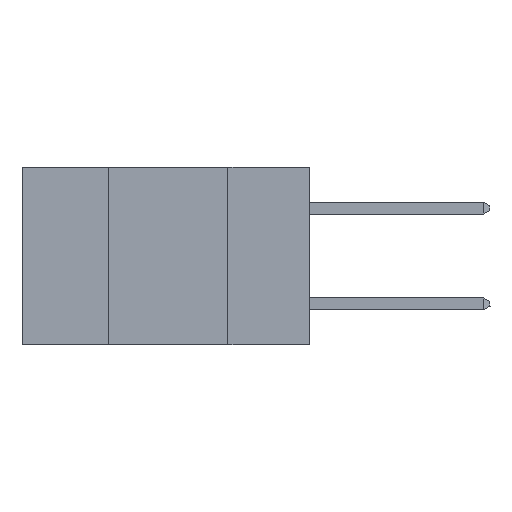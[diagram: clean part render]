
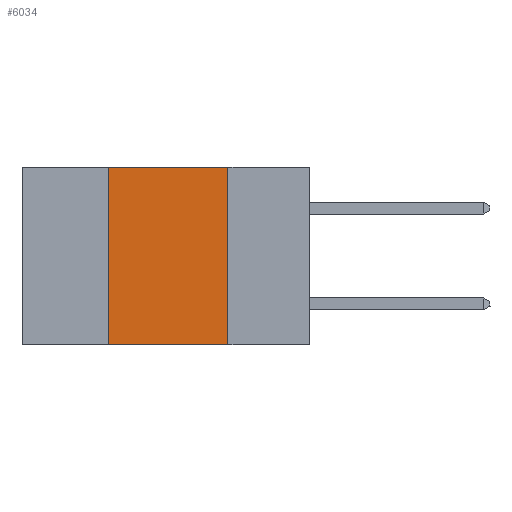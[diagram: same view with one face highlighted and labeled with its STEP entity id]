
A CAD part, left-side view. The second image highlights one B-rep face of the part: STEP entity #6034.
In plain terms, the highlighted planar face has unit normal (-1, 0, 0).
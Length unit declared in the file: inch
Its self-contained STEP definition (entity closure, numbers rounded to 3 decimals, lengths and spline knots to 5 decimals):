
#77 = ORIENTED_EDGE ( 'NONE', *, *, #10227, .F. ) ;
#319 = LINE ( 'NONE', #8412, #8513 ) ;
#782 = ORIENTED_EDGE ( 'NONE', *, *, #11418, .F. ) ;
#1010 = LINE ( 'NONE', #1358, #8605 ) ;
#1264 = ORIENTED_EDGE ( 'NONE', *, *, #11656, .T. ) ;
#1358 = CARTESIAN_POINT ( 'NONE',  ( 0., 0.6, 0. ) ) ;
#2071 = DIRECTION ( 'NONE',  ( 1., 0., 0. ) ) ;
#2886 = VERTEX_POINT ( 'NONE', #10582 ) ;
#3090 = VECTOR ( 'NONE', #4858, 39.37008 ) ;
#3802 = CARTESIAN_POINT ( 'NONE',  ( 0., 0.6, -0.37 ) ) ;
#4628 = DIRECTION ( 'NONE',  ( 0., -1., 0. ) ) ;
#4858 = DIRECTION ( 'NONE',  ( 0., -1., 0. ) ) ;
#5360 = CARTESIAN_POINT ( 'NONE',  ( 0., 0.17, -0.37 ) ) ;
#5440 = VERTEX_POINT ( 'NONE', #11956 ) ;
#5455 = EDGE_LOOP ( 'NONE', ( #6167, #77, #782, #1264 ) ) ;
#5644 = LINE ( 'NONE', #12753, #10733 ) ;
#5914 = EDGE_CURVE ( 'NONE', #5440, #10719, #5644, .T. ) ;
#6034 = ADVANCED_FACE ( 'NONE', ( #9893 ), #8161, .F. ) ;
#6167 = ORIENTED_EDGE ( 'NONE', *, *, #5914, .F. ) ;
#6242 = AXIS2_PLACEMENT_3D ( 'NONE', #11887, #2071, #9150 ) ;
#7051 = DIRECTION ( 'NONE',  ( 0., 0., -1. ) ) ;
#8161 = PLANE ( 'NONE',  #6242 ) ;
#8412 = CARTESIAN_POINT ( 'NONE',  ( 0., 0.42, 0. ) ) ;
#8513 = VECTOR ( 'NONE', #10314, 39.37008 ) ;
#8605 = VECTOR ( 'NONE', #4628, 39.37008 ) ;
#8619 = CARTESIAN_POINT ( 'NONE',  ( 0., 0.42, -0.37 ) ) ;
#9150 = DIRECTION ( 'NONE',  ( 0., 0., -1. ) ) ;
#9893 = FACE_OUTER_BOUND ( 'NONE', #5455, .T. ) ;
#10227 = EDGE_CURVE ( 'NONE', #2886, #5440, #1010, .T. ) ;
#10314 = DIRECTION ( 'NONE',  ( 0., 0., 1. ) ) ;
#10582 = CARTESIAN_POINT ( 'NONE',  ( 0., 0.42, 0. ) ) ;
#10622 = LINE ( 'NONE', #3802, #3090 ) ;
#10719 = VERTEX_POINT ( 'NONE', #5360 ) ;
#10733 = VECTOR ( 'NONE', #7051, 39.37008 ) ;
#11418 = EDGE_CURVE ( 'NONE', #11575, #2886, #319, .T. ) ;
#11575 = VERTEX_POINT ( 'NONE', #8619 ) ;
#11656 = EDGE_CURVE ( 'NONE', #11575, #10719, #10622, .T. ) ;
#11887 = CARTESIAN_POINT ( 'NONE',  ( 0., 0.6, 0. ) ) ;
#11956 = CARTESIAN_POINT ( 'NONE',  ( 0., 0.17, 0. ) ) ;
#12753 = CARTESIAN_POINT ( 'NONE',  ( 0., 0.17, 0. ) ) ;
